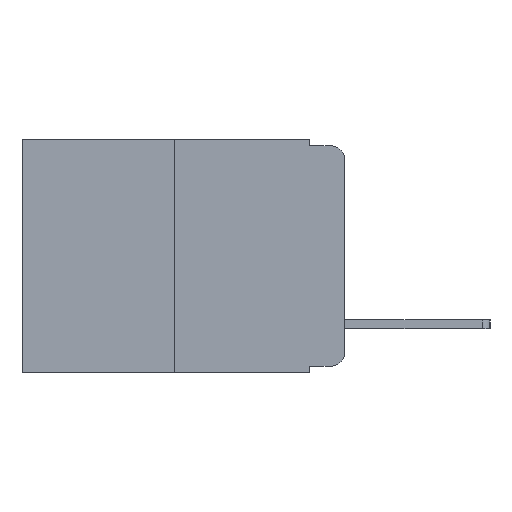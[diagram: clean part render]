
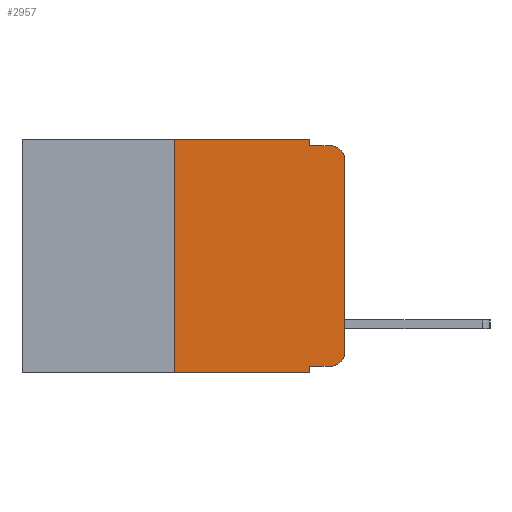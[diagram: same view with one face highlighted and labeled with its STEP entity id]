
A CAD part, left-side view. The second image highlights one B-rep face of the part: STEP entity #2957.
In plain terms, the highlighted planar face has unit normal (-1, 0, 0).
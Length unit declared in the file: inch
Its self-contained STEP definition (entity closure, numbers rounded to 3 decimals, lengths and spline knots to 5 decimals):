
#218 = ORIENTED_EDGE ( 'NONE', *, *, #11819, .T. ) ;
#252 = VECTOR ( 'NONE', #15883, 39.37008 ) ;
#313 = CARTESIAN_POINT ( 'NONE',  ( 0., 0.473, 0. ) ) ;
#363 = EDGE_LOOP ( 'NONE', ( #4838, #2536, #6045, #3763, #8566, #13633, #2136, #596, #4113, #218 ) ) ;
#484 = VECTOR ( 'NONE', #18877, 39.37008 ) ;
#596 = ORIENTED_EDGE ( 'NONE', *, *, #6601, .F. ) ;
#652 = CARTESIAN_POINT ( 'NONE',  ( 0., 0.051, -0.01 ) ) ;
#759 = CARTESIAN_POINT ( 'NONE',  ( 0., 0.02, -0.313 ) ) ;
#778 = CARTESIAN_POINT ( 'NONE',  ( 0., 0.051, -0.343 ) ) ;
#815 = CARTESIAN_POINT ( 'NONE',  ( 0., 0.25, 0. ) ) ;
#858 = EDGE_CURVE ( 'NONE', #10054, #8708, #18489, .T. ) ;
#1097 = PLANE ( 'NONE',  #17427 ) ;
#1153 = DIRECTION ( 'NONE',  ( 0., 0., 1. ) ) ;
#1646 = CIRCLE ( 'NONE', #15823, 0.02 ) ;
#2136 = ORIENTED_EDGE ( 'NONE', *, *, #15772, .T. ) ;
#2410 = DIRECTION ( 'NONE',  ( 0., 0., -1. ) ) ;
#2452 = CARTESIAN_POINT ( 'NONE',  ( 0., 0.25, -0.343 ) ) ;
#2536 = ORIENTED_EDGE ( 'NONE', *, *, #12063, .T. ) ;
#2957 = ADVANCED_FACE ( 'NONE', ( #11044 ), #1097, .F. ) ;
#3451 = EDGE_CURVE ( 'NONE', #6270, #19122, #4741, .T. ) ;
#3758 = CARTESIAN_POINT ( 'NONE',  ( 0., 0.02, -0.01 ) ) ;
#3763 = ORIENTED_EDGE ( 'NONE', *, *, #16276, .F. ) ;
#3890 = CARTESIAN_POINT ( 'NONE',  ( 0., 0., -0.313 ) ) ;
#4113 = ORIENTED_EDGE ( 'NONE', *, *, #3451, .T. ) ;
#4320 = CARTESIAN_POINT ( 'NONE',  ( 0., 0., 0. ) ) ;
#4328 = DIRECTION ( 'NONE',  ( 0., 0., -1. ) ) ;
#4741 = LINE ( 'NONE', #8815, #484 ) ;
#4838 = ORIENTED_EDGE ( 'NONE', *, *, #16896, .T. ) ;
#5324 = CARTESIAN_POINT ( 'NONE',  ( 0., 0., -0.03 ) ) ;
#5698 = AXIS2_PLACEMENT_3D ( 'NONE', #16189, #7558, #17650 ) ;
#6045 = ORIENTED_EDGE ( 'NONE', *, *, #858, .F. ) ;
#6083 = VERTEX_POINT ( 'NONE', #778 ) ;
#6142 = CARTESIAN_POINT ( 'NONE',  ( 0., 0.473, -0.343 ) ) ;
#6270 = VERTEX_POINT ( 'NONE', #17859 ) ;
#6466 = CARTESIAN_POINT ( 'NONE',  ( 0., 0.02, -0.333 ) ) ;
#6584 = VECTOR ( 'NONE', #17379, 39.37008 ) ;
#6601 = EDGE_CURVE ( 'NONE', #6270, #6083, #14310, .T. ) ;
#7047 = VECTOR ( 'NONE', #13493, 39.37008 ) ;
#7558 = DIRECTION ( 'NONE',  ( -1., 0., 0. ) ) ;
#7759 = EDGE_CURVE ( 'NONE', #18077, #16550, #18290, .T. ) ;
#8307 = VECTOR ( 'NONE', #1153, 39.37008 ) ;
#8566 = ORIENTED_EDGE ( 'NONE', *, *, #7759, .F. ) ;
#8583 = DIRECTION ( 'NONE',  ( 0., 0., 1. ) ) ;
#8708 = VERTEX_POINT ( 'NONE', #3758 ) ;
#8792 = VERTEX_POINT ( 'NONE', #3890 ) ;
#8815 = CARTESIAN_POINT ( 'NONE',  ( 0., 0.051, -0.333 ) ) ;
#9007 = LINE ( 'NONE', #13034, #252 ) ;
#9530 = EDGE_CURVE ( 'NONE', #14370, #18077, #14868, .T. ) ;
#10034 = CIRCLE ( 'NONE', #5698, 0.02 ) ;
#10054 = VERTEX_POINT ( 'NONE', #14489 ) ;
#10223 = CARTESIAN_POINT ( 'NONE',  ( 0., 0.473, 0. ) ) ;
#10897 = LINE ( 'NONE', #6142, #7047 ) ;
#11034 = DIRECTION ( 'NONE',  ( 0., -1., 0. ) ) ;
#11044 = FACE_OUTER_BOUND ( 'NONE', #363, .T. ) ;
#11429 = DIRECTION ( 'NONE',  ( -1., 0., 0. ) ) ;
#11640 = CARTESIAN_POINT ( 'NONE',  ( 0., 0.051, 0. ) ) ;
#11819 = EDGE_CURVE ( 'NONE', #19122, #8792, #1646, .T. ) ;
#12063 = EDGE_CURVE ( 'NONE', #17339, #8708, #10034, .T. ) ;
#13034 = CARTESIAN_POINT ( 'NONE',  ( 0., 0.051, 0. ) ) ;
#13226 = DIRECTION ( 'NONE',  ( 1., 0., 0. ) ) ;
#13493 = DIRECTION ( 'NONE',  ( 0., -1., 0. ) ) ;
#13633 = ORIENTED_EDGE ( 'NONE', *, *, #9530, .F. ) ;
#14175 = DIRECTION ( 'NONE',  ( 0., -1., 0. ) ) ;
#14310 = LINE ( 'NONE', #11640, #6584 ) ;
#14370 = VERTEX_POINT ( 'NONE', #2452 ) ;
#14489 = CARTESIAN_POINT ( 'NONE',  ( 0., 0.051, -0.01 ) ) ;
#14490 = VECTOR ( 'NONE', #11034, 39.37008 ) ;
#14675 = VECTOR ( 'NONE', #14175, 39.37008 ) ;
#14868 = LINE ( 'NONE', #815, #18677 ) ;
#15336 = CARTESIAN_POINT ( 'NONE',  ( 0., 0.051, 0. ) ) ;
#15772 = EDGE_CURVE ( 'NONE', #14370, #6083, #10897, .T. ) ;
#15823 = AXIS2_PLACEMENT_3D ( 'NONE', #759, #11429, #2410 ) ;
#15883 = DIRECTION ( 'NONE',  ( 0., 0., -1. ) ) ;
#15961 = LINE ( 'NONE', #4320, #8307 ) ;
#16189 = CARTESIAN_POINT ( 'NONE',  ( 0., 0.02, -0.03 ) ) ;
#16276 = EDGE_CURVE ( 'NONE', #16550, #10054, #9007, .T. ) ;
#16550 = VERTEX_POINT ( 'NONE', #15336 ) ;
#16896 = EDGE_CURVE ( 'NONE', #8792, #17339, #15961, .T. ) ;
#17339 = VERTEX_POINT ( 'NONE', #5324 ) ;
#17379 = DIRECTION ( 'NONE',  ( 0., 0., -1. ) ) ;
#17427 = AXIS2_PLACEMENT_3D ( 'NONE', #10223, #13226, #4328 ) ;
#17475 = CARTESIAN_POINT ( 'NONE',  ( 0., 0.25, 0. ) ) ;
#17650 = DIRECTION ( 'NONE',  ( 0., 0., -1. ) ) ;
#17859 = CARTESIAN_POINT ( 'NONE',  ( 0., 0.051, -0.333 ) ) ;
#18077 = VERTEX_POINT ( 'NONE', #17475 ) ;
#18290 = LINE ( 'NONE', #313, #14490 ) ;
#18489 = LINE ( 'NONE', #652, #14675 ) ;
#18677 = VECTOR ( 'NONE', #8583, 39.37008 ) ;
#18877 = DIRECTION ( 'NONE',  ( 0., -1., 0. ) ) ;
#19122 = VERTEX_POINT ( 'NONE', #6466 ) ;
